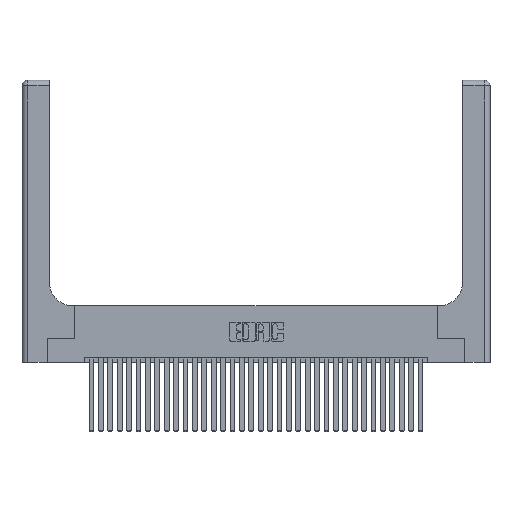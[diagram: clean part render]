
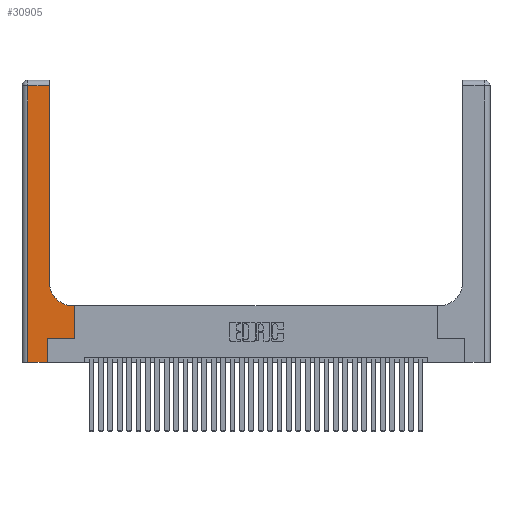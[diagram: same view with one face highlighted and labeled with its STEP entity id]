
A CAD part, top view. The second image highlights one B-rep face of the part: STEP entity #30905.
In plain terms, the highlighted planar face has unit normal (0, 0, 1).
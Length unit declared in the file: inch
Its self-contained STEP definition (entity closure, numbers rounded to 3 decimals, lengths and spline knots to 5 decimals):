
#438 = CARTESIAN_POINT ( 'NONE',  ( 0.269, 0.25, 0.37 ) ) ;
#980 = EDGE_CURVE ( 'NONE', #29465, #13084, #9359, .T. ) ;
#1366 = ORIENTED_EDGE ( 'NONE', *, *, #23179, .T. ) ;
#1729 = DIRECTION ( 'NONE',  ( 0., 1., 0. ) ) ;
#2139 = VERTEX_POINT ( 'NONE', #7220 ) ;
#2667 = LINE ( 'NONE', #23025, #22991 ) ;
#3747 = PLANE ( 'NONE',  #19033 ) ;
#3857 = DIRECTION ( 'NONE',  ( -1., 0., 0. ) ) ;
#4331 = CARTESIAN_POINT ( 'NONE',  ( 0.2915, 0.6, 0.37 ) ) ;
#4495 = DIRECTION ( 'NONE',  ( 1., 0., 0. ) ) ;
#4534 = VERTEX_POINT ( 'NONE', #19234 ) ;
#5938 = DIRECTION ( 'NONE',  ( 1., 0., 0. ) ) ;
#6096 = ORIENTED_EDGE ( 'NONE', *, *, #14092, .T. ) ;
#6521 = VECTOR ( 'NONE', #21023, 39.37008 ) ;
#6860 = CARTESIAN_POINT ( 'NONE',  ( 0.06, 3., 0.37 ) ) ;
#6930 = LINE ( 'NONE', #438, #26242 ) ;
#7220 = CARTESIAN_POINT ( 'NONE',  ( 0.5585, 0.25, 0.37 ) ) ;
#7741 = CARTESIAN_POINT ( 'NONE',  ( 0.5415, 0.6, 0.37 ) ) ;
#8425 = ORIENTED_EDGE ( 'NONE', *, *, #26801, .T. ) ;
#8846 = VERTEX_POINT ( 'NONE', #28119 ) ;
#8851 = VERTEX_POINT ( 'NONE', #12623 ) ;
#8966 = VECTOR ( 'NONE', #20564, 39.37008 ) ;
#9032 = EDGE_CURVE ( 'NONE', #12244, #17559, #2667, .T. ) ;
#9359 = CIRCLE ( 'NONE', #17950, 0.25 ) ;
#9685 = DIRECTION ( 'NONE',  ( 0., 0., -1. ) ) ;
#10112 = CARTESIAN_POINT ( 'NONE',  ( 0.2915, 3., 0.37 ) ) ;
#10585 = VECTOR ( 'NONE', #25851, 39.37008 ) ;
#11868 = EDGE_CURVE ( 'NONE', #8846, #12244, #23809, .T. ) ;
#11918 = CARTESIAN_POINT ( 'NONE',  ( 0., 3., 0.37 ) ) ;
#12244 = VERTEX_POINT ( 'NONE', #16596 ) ;
#12416 = EDGE_CURVE ( 'NONE', #17559, #32847, #16129, .T. ) ;
#12623 = CARTESIAN_POINT ( 'NONE',  ( 0.5585, 0.6, 0.37 ) ) ;
#13084 = VERTEX_POINT ( 'NONE', #33170 ) ;
#14092 = EDGE_CURVE ( 'NONE', #32847, #2139, #6930, .T. ) ;
#14453 = CARTESIAN_POINT ( 'NONE',  ( 0.269, 0., 0.37 ) ) ;
#15085 = DIRECTION ( 'NONE',  ( -1., 0., 0. ) ) ;
#16129 = LINE ( 'NONE', #28178, #8966 ) ;
#16596 = CARTESIAN_POINT ( 'NONE',  ( 0.06, 0., 0.37 ) ) ;
#17188 = ORIENTED_EDGE ( 'NONE', *, *, #9032, .T. ) ;
#17197 = EDGE_CURVE ( 'NONE', #13084, #4534, #18453, .T. ) ;
#17559 = VERTEX_POINT ( 'NONE', #14453 ) ;
#17950 = AXIS2_PLACEMENT_3D ( 'NONE', #25347, #9685, #27930 ) ;
#18312 = FACE_OUTER_BOUND ( 'NONE', #32653, .T. ) ;
#18453 = LINE ( 'NONE', #10112, #10585 ) ;
#19033 = AXIS2_PLACEMENT_3D ( 'NONE', #11918, #19837, #3857 ) ;
#19203 = ORIENTED_EDGE ( 'NONE', *, *, #32906, .T. ) ;
#19234 = CARTESIAN_POINT ( 'NONE',  ( 0.2915, 2.94, 0.37 ) ) ;
#19404 = LINE ( 'NONE', #4331, #26216 ) ;
#19837 = DIRECTION ( 'NONE',  ( 0., 0., -1. ) ) ;
#20121 = DIRECTION ( 'NONE',  ( 0., -1., 0. ) ) ;
#20564 = DIRECTION ( 'NONE',  ( 0., 1., 0. ) ) ;
#20912 = CARTESIAN_POINT ( 'NONE',  ( 0., 2.94, 0.37 ) ) ;
#21023 = DIRECTION ( 'NONE',  ( -1., 0., 0. ) ) ;
#21460 = ORIENTED_EDGE ( 'NONE', *, *, #12416, .T. ) ;
#21484 = LINE ( 'NONE', #20912, #6521 ) ;
#22952 = ORIENTED_EDGE ( 'NONE', *, *, #980, .T. ) ;
#22991 = VECTOR ( 'NONE', #4495, 39.37008 ) ;
#23025 = CARTESIAN_POINT ( 'NONE',  ( 0., 0., 0.37 ) ) ;
#23179 = EDGE_CURVE ( 'NONE', #2139, #8851, #24945, .T. ) ;
#23809 = LINE ( 'NONE', #6860, #30601 ) ;
#24159 = VECTOR ( 'NONE', #1729, 39.37008 ) ;
#24945 = LINE ( 'NONE', #28017, #24159 ) ;
#25222 = CARTESIAN_POINT ( 'NONE',  ( 0.269, 0.25, 0.37 ) ) ;
#25347 = CARTESIAN_POINT ( 'NONE',  ( 0.5415, 0.85, 0.37 ) ) ;
#25851 = DIRECTION ( 'NONE',  ( 0., 1., 0. ) ) ;
#26216 = VECTOR ( 'NONE', #15085, 39.37008 ) ;
#26242 = VECTOR ( 'NONE', #5938, 39.37008 ) ;
#26801 = EDGE_CURVE ( 'NONE', #4534, #8846, #21484, .T. ) ;
#27930 = DIRECTION ( 'NONE',  ( 1., 0., 0. ) ) ;
#28017 = CARTESIAN_POINT ( 'NONE',  ( 0.5585, 0.25, 0.37 ) ) ;
#28119 = CARTESIAN_POINT ( 'NONE',  ( 0.06, 2.94, 0.37 ) ) ;
#28178 = CARTESIAN_POINT ( 'NONE',  ( 0.269, 0., 0.37 ) ) ;
#28536 = ORIENTED_EDGE ( 'NONE', *, *, #17197, .T. ) ;
#29465 = VERTEX_POINT ( 'NONE', #7741 ) ;
#30601 = VECTOR ( 'NONE', #20121, 39.37008 ) ;
#30905 = ADVANCED_FACE ( 'NONE', ( #18312 ), #3747, .F. ) ;
#32653 = EDGE_LOOP ( 'NONE', ( #28536, #8425, #33621, #17188, #21460, #6096, #1366, #19203, #22952 ) ) ;
#32847 = VERTEX_POINT ( 'NONE', #25222 ) ;
#32906 = EDGE_CURVE ( 'NONE', #8851, #29465, #19404, .T. ) ;
#33170 = CARTESIAN_POINT ( 'NONE',  ( 0.2915, 0.85, 0.37 ) ) ;
#33621 = ORIENTED_EDGE ( 'NONE', *, *, #11868, .T. ) ;
